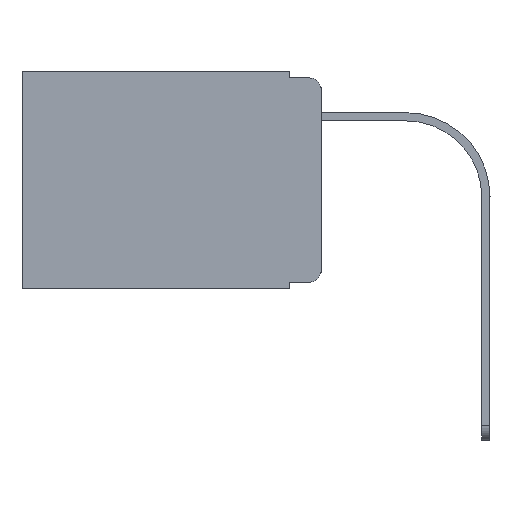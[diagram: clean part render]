
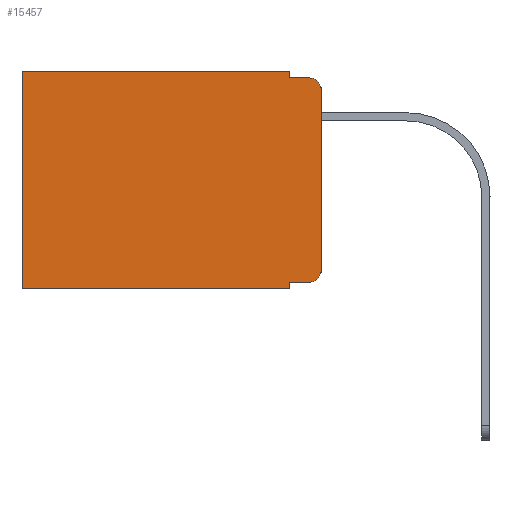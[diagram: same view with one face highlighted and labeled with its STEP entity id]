
A CAD part, left-side view. The second image highlights one B-rep face of the part: STEP entity #15457.
In plain terms, the highlighted planar face has unit normal (-1, 0, 0).
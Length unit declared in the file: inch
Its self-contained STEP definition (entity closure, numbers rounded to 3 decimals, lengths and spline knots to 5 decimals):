
#52 = VERTEX_POINT ( 'NONE', #4779 ) ;
#330 = VERTEX_POINT ( 'NONE', #6640 ) ;
#409 = EDGE_CURVE ( 'NONE', #9978, #11470, #13450, .T. ) ;
#815 = CARTESIAN_POINT ( 'NONE',  ( 0.298, 0.02, -0.03 ) ) ;
#909 = EDGE_CURVE ( 'NONE', #9978, #16627, #14863, .T. ) ;
#1316 = DIRECTION ( 'NONE',  ( 0., 0., -1. ) ) ;
#1442 = FACE_OUTER_BOUND ( 'NONE', #2517, .T. ) ;
#1490 = VERTEX_POINT ( 'NONE', #3931 ) ;
#1782 = VECTOR ( 'NONE', #15943, 39.37008 ) ;
#1793 = DIRECTION ( 'NONE',  ( 1., 0., 0. ) ) ;
#2391 = DIRECTION ( 'NONE',  ( 0., 0., -1. ) ) ;
#2411 = CARTESIAN_POINT ( 'NONE',  ( 0.298, 0.051, 0. ) ) ;
#2517 = EDGE_LOOP ( 'NONE', ( #15458, #9759, #11159, #9537, #7670, #9833, #7844, #7279, #4143, #7734 ) ) ;
#2699 = DIRECTION ( 'NONE',  ( 0., 1., 0. ) ) ;
#3459 = AXIS2_PLACEMENT_3D ( 'NONE', #6842, #1793, #16316 ) ;
#3931 = CARTESIAN_POINT ( 'NONE',  ( 0.298, 0.051, -0.01 ) ) ;
#4143 = ORIENTED_EDGE ( 'NONE', *, *, #11104, .T. ) ;
#4552 = CARTESIAN_POINT ( 'NONE',  ( 0.298, 0.051, 0. ) ) ;
#4779 = CARTESIAN_POINT ( 'NONE',  ( 0.298, 0.051, 0. ) ) ;
#4876 = DIRECTION ( 'NONE',  ( 0., 0., -1. ) ) ;
#4971 = EDGE_CURVE ( 'NONE', #12157, #16627, #16006, .T. ) ;
#5381 = CARTESIAN_POINT ( 'NONE',  ( 0.298, 0., -0.343 ) ) ;
#5569 = VERTEX_POINT ( 'NONE', #11923 ) ;
#6021 = VECTOR ( 'NONE', #8006, 39.37008 ) ;
#6233 = VERTEX_POINT ( 'NONE', #14439 ) ;
#6299 = LINE ( 'NONE', #11708, #8675 ) ;
#6562 = DIRECTION ( 'NONE',  ( 0., -1., 0. ) ) ;
#6640 = CARTESIAN_POINT ( 'NONE',  ( 0.298, 0.051, -0.343 ) ) ;
#6842 = CARTESIAN_POINT ( 'NONE',  ( 0.298, 0., 0. ) ) ;
#7129 = CARTESIAN_POINT ( 'NONE',  ( 0.298, 0.02, -0.333 ) ) ;
#7279 = ORIENTED_EDGE ( 'NONE', *, *, #15777, .F. ) ;
#7371 = LINE ( 'NONE', #10134, #8733 ) ;
#7386 = EDGE_CURVE ( 'NONE', #1490, #11470, #7371, .T. ) ;
#7585 = LINE ( 'NONE', #4552, #13118 ) ;
#7670 = ORIENTED_EDGE ( 'NONE', *, *, #12572, .T. ) ;
#7734 = ORIENTED_EDGE ( 'NONE', *, *, #4971, .T. ) ;
#7844 = ORIENTED_EDGE ( 'NONE', *, *, #13340, .F. ) ;
#7881 = CARTESIAN_POINT ( 'NONE',  ( 0.298, 0., 0. ) ) ;
#7965 = DIRECTION ( 'NONE',  ( 0., 1., 0. ) ) ;
#8006 = DIRECTION ( 'NONE',  ( 0., -1., 0. ) ) ;
#8611 = CARTESIAN_POINT ( 'NONE',  ( 0.298, 0.02, -0.01 ) ) ;
#8675 = VECTOR ( 'NONE', #4876, 39.37008 ) ;
#8733 = VECTOR ( 'NONE', #6562, 39.37008 ) ;
#8770 = CARTESIAN_POINT ( 'NONE',  ( 0.298, 0.051, -0.333 ) ) ;
#8969 = DIRECTION ( 'NONE',  ( -1., 0., 0. ) ) ;
#9039 = VERTEX_POINT ( 'NONE', #8770 ) ;
#9537 = ORIENTED_EDGE ( 'NONE', *, *, #9679, .F. ) ;
#9679 = EDGE_CURVE ( 'NONE', #52, #1490, #7585, .T. ) ;
#9759 = ORIENTED_EDGE ( 'NONE', *, *, #409, .T. ) ;
#9833 = ORIENTED_EDGE ( 'NONE', *, *, #14061, .T. ) ;
#9864 = PLANE ( 'NONE',  #3459 ) ;
#9978 = VERTEX_POINT ( 'NONE', #14922 ) ;
#10134 = CARTESIAN_POINT ( 'NONE',  ( 0.298, 0.051, -0.01 ) ) ;
#10347 = CARTESIAN_POINT ( 'NONE',  ( 0.298, 0., -0.313 ) ) ;
#11104 = EDGE_CURVE ( 'NONE', #9039, #12157, #12078, .T. ) ;
#11159 = ORIENTED_EDGE ( 'NONE', *, *, #7386, .F. ) ;
#11470 = VERTEX_POINT ( 'NONE', #8611 ) ;
#11708 = CARTESIAN_POINT ( 'NONE',  ( 0.298, 0.473, 0. ) ) ;
#11861 = DIRECTION ( 'NONE',  ( -1., 0., 0. ) ) ;
#11923 = CARTESIAN_POINT ( 'NONE',  ( 0.298, 0.473, 0. ) ) ;
#12073 = VECTOR ( 'NONE', #1316, 39.37008 ) ;
#12078 = LINE ( 'NONE', #14557, #6021 ) ;
#12157 = VERTEX_POINT ( 'NONE', #7129 ) ;
#12572 = EDGE_CURVE ( 'NONE', #52, #5569, #13327, .T. ) ;
#12857 = CARTESIAN_POINT ( 'NONE',  ( 0.298, 0.02, -0.313 ) ) ;
#13118 = VECTOR ( 'NONE', #16758, 39.37008 ) ;
#13160 = VECTOR ( 'NONE', #2699, 39.37008 ) ;
#13327 = LINE ( 'NONE', #14818, #13160 ) ;
#13340 = EDGE_CURVE ( 'NONE', #330, #6233, #14765, .T. ) ;
#13450 = CIRCLE ( 'NONE', #17379, 0.02 ) ;
#14061 = EDGE_CURVE ( 'NONE', #5569, #6233, #6299, .T. ) ;
#14377 = DIRECTION ( 'NONE',  ( 0., 0., -1. ) ) ;
#14439 = CARTESIAN_POINT ( 'NONE',  ( 0.298, 0.473, -0.343 ) ) ;
#14557 = CARTESIAN_POINT ( 'NONE',  ( 0.298, 0.051, -0.333 ) ) ;
#14765 = LINE ( 'NONE', #5381, #16837 ) ;
#14818 = CARTESIAN_POINT ( 'NONE',  ( 0.298, 0., 0. ) ) ;
#14863 = LINE ( 'NONE', #7881, #12073 ) ;
#14922 = CARTESIAN_POINT ( 'NONE',  ( 0.298, 0., -0.03 ) ) ;
#15457 = ADVANCED_FACE ( 'NONE', ( #1442 ), #9864, .F. ) ;
#15458 = ORIENTED_EDGE ( 'NONE', *, *, #909, .F. ) ;
#15713 = AXIS2_PLACEMENT_3D ( 'NONE', #12857, #11861, #2391 ) ;
#15777 = EDGE_CURVE ( 'NONE', #9039, #330, #16121, .T. ) ;
#15943 = DIRECTION ( 'NONE',  ( 0., 0., -1. ) ) ;
#16006 = CIRCLE ( 'NONE', #15713, 0.02 ) ;
#16121 = LINE ( 'NONE', #2411, #1782 ) ;
#16316 = DIRECTION ( 'NONE',  ( 0., 0., -1. ) ) ;
#16627 = VERTEX_POINT ( 'NONE', #10347 ) ;
#16758 = DIRECTION ( 'NONE',  ( 0., 0., -1. ) ) ;
#16837 = VECTOR ( 'NONE', #7965, 39.37008 ) ;
#17379 = AXIS2_PLACEMENT_3D ( 'NONE', #815, #8969, #14377 ) ;
